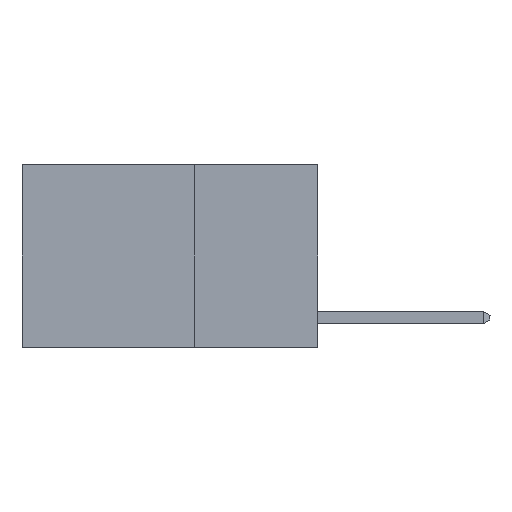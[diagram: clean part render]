
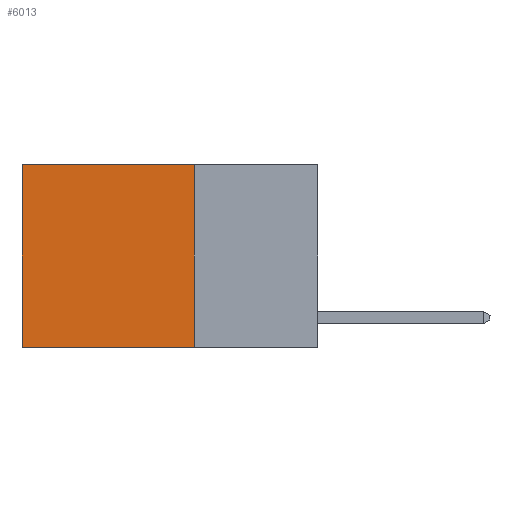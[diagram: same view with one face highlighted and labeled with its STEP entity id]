
A CAD part, left-side view. The second image highlights one B-rep face of the part: STEP entity #6013.
In plain terms, the highlighted planar face has unit normal (-1, 0, 0).
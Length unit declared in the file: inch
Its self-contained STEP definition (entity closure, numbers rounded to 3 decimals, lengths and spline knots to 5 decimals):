
#409 = CARTESIAN_POINT ( 'NONE',  ( 0.2625, 0.25, 0. ) ) ;
#1121 = LINE ( 'NONE', #3197, #11095 ) ;
#1337 = CARTESIAN_POINT ( 'NONE',  ( 0.2625, 0.25, 0. ) ) ;
#1718 = VECTOR ( 'NONE', #13838, 39.37008 ) ;
#1746 = DIRECTION ( 'NONE',  ( 0., 1., 0. ) ) ;
#3197 = CARTESIAN_POINT ( 'NONE',  ( 0.2625, 0.25, 0. ) ) ;
#3221 = DIRECTION ( 'NONE',  ( 0., 1., 0. ) ) ;
#3398 = LINE ( 'NONE', #409, #9839 ) ;
#4171 = VECTOR ( 'NONE', #3221, 39.37008 ) ;
#4496 = AXIS2_PLACEMENT_3D ( 'NONE', #1337, #15703, #7952 ) ;
#4872 = EDGE_LOOP ( 'NONE', ( #4929, #5849, #13779, #8317 ) ) ;
#4929 = ORIENTED_EDGE ( 'NONE', *, *, #14574, .T. ) ;
#5849 = ORIENTED_EDGE ( 'NONE', *, *, #15725, .F. ) ;
#6013 = ADVANCED_FACE ( 'NONE', ( #11416 ), #6690, .F. ) ;
#6690 = PLANE ( 'NONE',  #4496 ) ;
#6841 = VERTEX_POINT ( 'NONE', #11097 ) ;
#7952 = DIRECTION ( 'NONE',  ( 0., 0., -1. ) ) ;
#8317 = ORIENTED_EDGE ( 'NONE', *, *, #9000, .T. ) ;
#8638 = LINE ( 'NONE', #15071, #1718 ) ;
#9000 = EDGE_CURVE ( 'NONE', #15012, #14056, #3398, .T. ) ;
#9839 = VECTOR ( 'NONE', #1746, 39.37008 ) ;
#10746 = CARTESIAN_POINT ( 'NONE',  ( 0.2625, 0.25, 0. ) ) ;
#11095 = VECTOR ( 'NONE', #13602, 39.37008 ) ;
#11097 = CARTESIAN_POINT ( 'NONE',  ( 0.2625, 0.25, -0.37 ) ) ;
#11416 = FACE_OUTER_BOUND ( 'NONE', #4872, .T. ) ;
#12241 = CARTESIAN_POINT ( 'NONE',  ( 0.2625, 0.25, -0.37 ) ) ;
#12835 = EDGE_CURVE ( 'NONE', #15012, #6841, #1121, .T. ) ;
#13456 = CARTESIAN_POINT ( 'NONE',  ( 0.2625, 0.6, -0.37 ) ) ;
#13602 = DIRECTION ( 'NONE',  ( 0., 0., -1. ) ) ;
#13779 = ORIENTED_EDGE ( 'NONE', *, *, #12835, .F. ) ;
#13838 = DIRECTION ( 'NONE',  ( 0., 0., -1. ) ) ;
#14056 = VERTEX_POINT ( 'NONE', #16600 ) ;
#14487 = LINE ( 'NONE', #12241, #4171 ) ;
#14574 = EDGE_CURVE ( 'NONE', #14056, #15669, #8638, .T. ) ;
#15012 = VERTEX_POINT ( 'NONE', #10746 ) ;
#15071 = CARTESIAN_POINT ( 'NONE',  ( 0.2625, 0.6, 0. ) ) ;
#15669 = VERTEX_POINT ( 'NONE', #13456 ) ;
#15703 = DIRECTION ( 'NONE',  ( 1., 0., 0. ) ) ;
#15725 = EDGE_CURVE ( 'NONE', #6841, #15669, #14487, .T. ) ;
#16600 = CARTESIAN_POINT ( 'NONE',  ( 0.2625, 0.6, 0. ) ) ;
